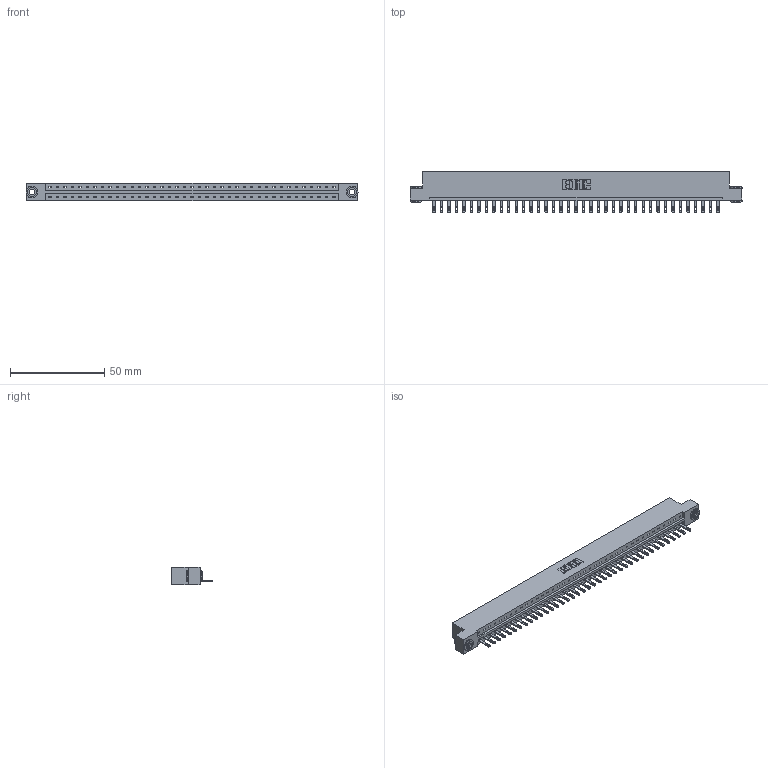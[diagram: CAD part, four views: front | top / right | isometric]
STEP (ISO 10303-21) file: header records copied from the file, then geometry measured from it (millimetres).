
FILE_DESCRIPTION (( 'STEP AP203' ), '1' );
FILE_NAME ('333-039-500-103.STEP', '2018-08-03T12:22:21', ( '' ), ( '' ), 'SwSTEP 2.0', 'SolidWorks 2016', '' );
FILE_SCHEMA (( 'CONFIG_CONTROL_DESIGN' ));
Length unit declared in the file: inch
Products named in the file (4): 333-039-500-103; 333 Part_Flush - .156 Dia - TH; 345-292-001_345-293-100; 345-250-002_345-250-002-102
Assembly tree (42 placements, depth 2):
  333-039-500-103
    333 Part_Flush - .156 Dia - TH
    345-292-001_345-293-100  x39
    345-250-002_345-250-002-102  x2
Bounding box: 176.07 x 21.85 x 9.4 mm (x, y, z)
Volume: 17735.6 mm3; surface area: 19492.3 mm2
Topology: 42 solids, 42 shells, 2258 faces, 6939 edges, 4622 vertices
Faces by surface type: plane 1484, cylinder 766, cone 8
Entity records: 24810 total; most frequent: CARTESIAN_POINT 4258, ORIENTED_EDGE 4226, DIRECTION 3633, EDGE_CURVE 2113, VECTOR 1957, LINE 1957, VERTEX_POINT 1406, AXIS2_PLACEMENT_3D 838
